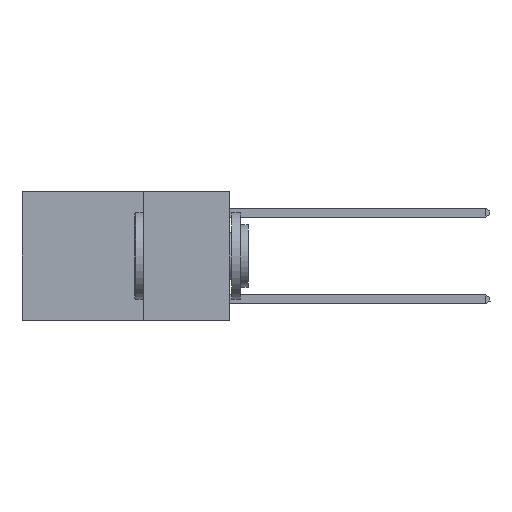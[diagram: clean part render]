
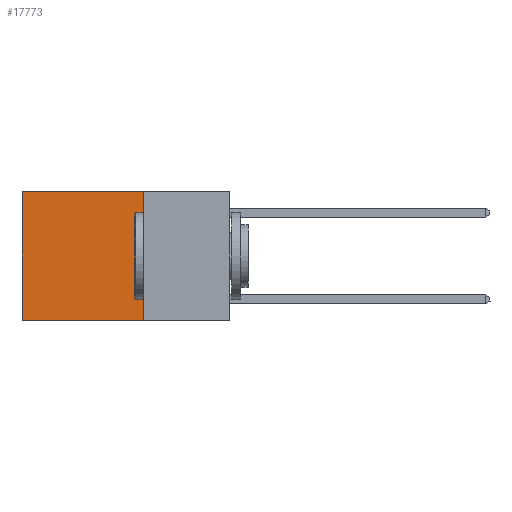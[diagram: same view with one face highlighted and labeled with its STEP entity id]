
A CAD part, left-side view. The second image highlights one B-rep face of the part: STEP entity #17773.
In plain terms, the highlighted planar face has unit normal (-1, 0, 0).
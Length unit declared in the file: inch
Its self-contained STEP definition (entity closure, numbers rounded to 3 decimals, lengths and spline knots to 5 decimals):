
#309 = VECTOR ( 'NONE', #6199, 39.37008 ) ;
#608 = CARTESIAN_POINT ( 'NONE',  ( 0.2625, 0.6, 0. ) ) ;
#1569 = EDGE_CURVE ( 'NONE', #11385, #16684, #12044, .T. ) ;
#1907 = DIRECTION ( 'NONE',  ( 0., 0., -1. ) ) ;
#2039 = CARTESIAN_POINT ( 'NONE',  ( 0.2625, 0.25, 0. ) ) ;
#2048 = LINE ( 'NONE', #17597, #18263 ) ;
#2246 = DIRECTION ( 'NONE',  ( 0., 0., -1. ) ) ;
#2383 = EDGE_CURVE ( 'NONE', #11764, #16684, #15411, .T. ) ;
#5536 = CARTESIAN_POINT ( 'NONE',  ( 0.2625, 0.25, 0. ) ) ;
#5552 = FACE_OUTER_BOUND ( 'NONE', #14275, .T. ) ;
#6199 = DIRECTION ( 'NONE',  ( 0., 1., 0. ) ) ;
#6520 = ORIENTED_EDGE ( 'NONE', *, *, #2383, .T. ) ;
#6913 = CARTESIAN_POINT ( 'NONE',  ( 0.2625, 0.25, -0.37 ) ) ;
#7091 = VECTOR ( 'NONE', #2246, 39.37008 ) ;
#8236 = EDGE_CURVE ( 'NONE', #16137, #11764, #9849, .T. ) ;
#8456 = CARTESIAN_POINT ( 'NONE',  ( 0.2625, 0.6, 0. ) ) ;
#9849 = LINE ( 'NONE', #2039, #17602 ) ;
#10083 = EDGE_CURVE ( 'NONE', #16137, #11385, #2048, .T. ) ;
#10340 = DIRECTION ( 'NONE',  ( 0., 0., -1. ) ) ;
#11385 = VERTEX_POINT ( 'NONE', #12311 ) ;
#11764 = VERTEX_POINT ( 'NONE', #8456 ) ;
#12044 = LINE ( 'NONE', #6913, #309 ) ;
#12311 = CARTESIAN_POINT ( 'NONE',  ( 0.2625, 0.25, -0.37 ) ) ;
#12428 = AXIS2_PLACEMENT_3D ( 'NONE', #5536, #19556, #10340 ) ;
#12506 = ORIENTED_EDGE ( 'NONE', *, *, #8236, .T. ) ;
#12508 = CARTESIAN_POINT ( 'NONE',  ( 0.2625, 0.6, -0.37 ) ) ;
#13114 = ORIENTED_EDGE ( 'NONE', *, *, #1569, .F. ) ;
#13138 = DIRECTION ( 'NONE',  ( 0., 1., 0. ) ) ;
#13402 = PLANE ( 'NONE',  #12428 ) ;
#14275 = EDGE_LOOP ( 'NONE', ( #6520, #13114, #15993, #12506 ) ) ;
#15411 = LINE ( 'NONE', #608, #7091 ) ;
#15993 = ORIENTED_EDGE ( 'NONE', *, *, #10083, .F. ) ;
#16137 = VERTEX_POINT ( 'NONE', #18882 ) ;
#16684 = VERTEX_POINT ( 'NONE', #12508 ) ;
#17597 = CARTESIAN_POINT ( 'NONE',  ( 0.2625, 0.25, 0. ) ) ;
#17602 = VECTOR ( 'NONE', #13138, 39.37008 ) ;
#17773 = ADVANCED_FACE ( 'NONE', ( #5552 ), #13402, .F. ) ;
#18263 = VECTOR ( 'NONE', #1907, 39.37008 ) ;
#18882 = CARTESIAN_POINT ( 'NONE',  ( 0.2625, 0.25, 0. ) ) ;
#19556 = DIRECTION ( 'NONE',  ( 1., 0., 0. ) ) ;
